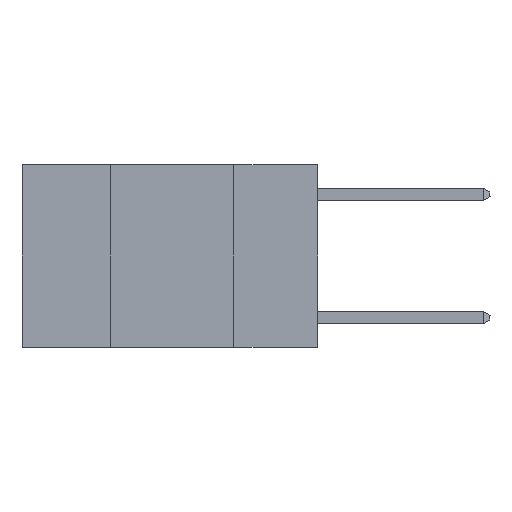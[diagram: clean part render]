
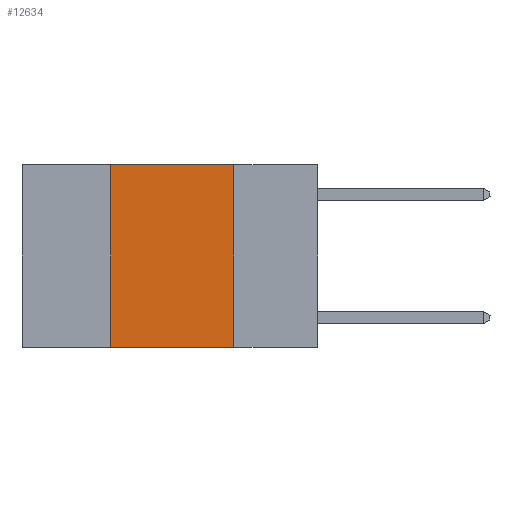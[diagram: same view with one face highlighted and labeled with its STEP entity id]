
A CAD part, left-side view. The second image highlights one B-rep face of the part: STEP entity #12634.
In plain terms, the highlighted planar face has unit normal (-1, 0, 0).
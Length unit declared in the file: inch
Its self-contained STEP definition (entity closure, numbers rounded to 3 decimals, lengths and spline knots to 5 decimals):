
#784 = ORIENTED_EDGE ( 'NONE', *, *, #9002, .F. ) ;
#859 = DIRECTION ( 'NONE',  ( 0., -1., 0. ) ) ;
#1330 = LINE ( 'NONE', #13182, #13515 ) ;
#1355 = DIRECTION ( 'NONE',  ( 1., 0., 0. ) ) ;
#1907 = DIRECTION ( 'NONE',  ( 0., 0., -1. ) ) ;
#2245 = LINE ( 'NONE', #7609, #6160 ) ;
#3030 = EDGE_LOOP ( 'NONE', ( #13705, #11339, #784, #5144 ) ) ;
#3729 = FACE_OUTER_BOUND ( 'NONE', #3030, .T. ) ;
#3941 = CARTESIAN_POINT ( 'NONE',  ( 0., 0.42, -0.37 ) ) ;
#3993 = CARTESIAN_POINT ( 'NONE',  ( 0., 0.17, 0. ) ) ;
#4016 = DIRECTION ( 'NONE',  ( 0., 0., 1. ) ) ;
#4510 = EDGE_CURVE ( 'NONE', #15607, #7619, #16572, .T. ) ;
#5144 = ORIENTED_EDGE ( 'NONE', *, *, #15503, .T. ) ;
#6039 = CARTESIAN_POINT ( 'NONE',  ( 0., 0.17, 0. ) ) ;
#6160 = VECTOR ( 'NONE', #12958, 39.37008 ) ;
#6340 = VERTEX_POINT ( 'NONE', #12428 ) ;
#7609 = CARTESIAN_POINT ( 'NONE',  ( 0., 0.6, -0.37 ) ) ;
#7619 = VERTEX_POINT ( 'NONE', #9289 ) ;
#7688 = DIRECTION ( 'NONE',  ( 0., 0., -1. ) ) ;
#8393 = LINE ( 'NONE', #13745, #8532 ) ;
#8532 = VECTOR ( 'NONE', #4016, 39.37008 ) ;
#8559 = EDGE_CURVE ( 'NONE', #6340, #15607, #1330, .T. ) ;
#8649 = AXIS2_PLACEMENT_3D ( 'NONE', #9107, #1355, #7688 ) ;
#9002 = EDGE_CURVE ( 'NONE', #10325, #6340, #8393, .T. ) ;
#9107 = CARTESIAN_POINT ( 'NONE',  ( 0., 0.6, 0. ) ) ;
#9289 = CARTESIAN_POINT ( 'NONE',  ( 0., 0.17, -0.37 ) ) ;
#10325 = VERTEX_POINT ( 'NONE', #3941 ) ;
#11339 = ORIENTED_EDGE ( 'NONE', *, *, #8559, .F. ) ;
#11503 = VECTOR ( 'NONE', #1907, 39.37008 ) ;
#12428 = CARTESIAN_POINT ( 'NONE',  ( 0., 0.42, 0. ) ) ;
#12634 = ADVANCED_FACE ( 'NONE', ( #3729 ), #17109, .F. ) ;
#12958 = DIRECTION ( 'NONE',  ( 0., -1., 0. ) ) ;
#13182 = CARTESIAN_POINT ( 'NONE',  ( 0., 0.6, 0. ) ) ;
#13515 = VECTOR ( 'NONE', #859, 39.37008 ) ;
#13705 = ORIENTED_EDGE ( 'NONE', *, *, #4510, .F. ) ;
#13745 = CARTESIAN_POINT ( 'NONE',  ( 0., 0.42, 0. ) ) ;
#15503 = EDGE_CURVE ( 'NONE', #10325, #7619, #2245, .T. ) ;
#15607 = VERTEX_POINT ( 'NONE', #3993 ) ;
#16572 = LINE ( 'NONE', #6039, #11503 ) ;
#17109 = PLANE ( 'NONE',  #8649 ) ;
